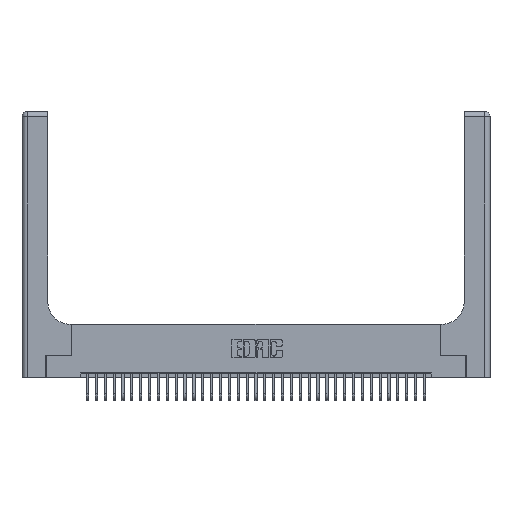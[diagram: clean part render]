
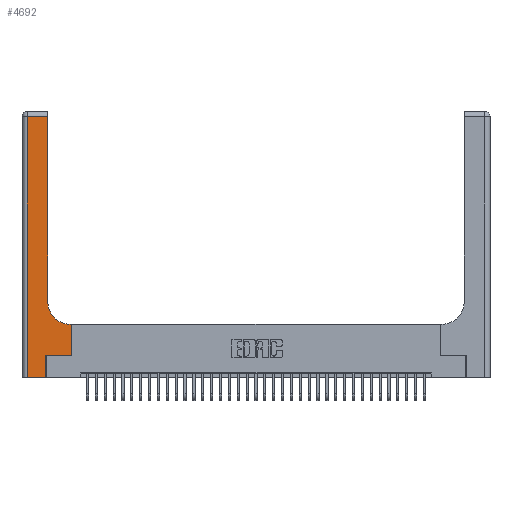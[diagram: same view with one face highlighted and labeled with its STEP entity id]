
A CAD part, top view. The second image highlights one B-rep face of the part: STEP entity #4692.
In plain terms, the highlighted planar face has unit normal (0, 0, 1).
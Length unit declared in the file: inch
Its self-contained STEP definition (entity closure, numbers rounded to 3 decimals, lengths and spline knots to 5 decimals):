
#306 = EDGE_CURVE ( 'NONE', #33902, #18627, #34485, .T. ) ;
#442 = ORIENTED_EDGE ( 'NONE', *, *, #20824, .T. ) ;
#2268 = DIRECTION ( 'NONE',  ( 0., 0., -1. ) ) ;
#2276 = VECTOR ( 'NONE', #25158, 39.37008 ) ;
#3361 = EDGE_CURVE ( 'NONE', #24542, #6409, #11562, .T. ) ;
#4110 = EDGE_CURVE ( 'NONE', #6556, #35407, #18662, .T. ) ;
#4316 = EDGE_CURVE ( 'NONE', #35407, #33902, #12256, .T. ) ;
#4446 = EDGE_CURVE ( 'NONE', #15794, #24542, #24082, .T. ) ;
#4692 = ADVANCED_FACE ( 'NONE', ( #30439 ), #23582, .F. ) ;
#5081 = CARTESIAN_POINT ( 'NONE',  ( 0., 0., 0.37 ) ) ;
#5613 = CARTESIAN_POINT ( 'NONE',  ( 0.5585, 0.6, 0.37 ) ) ;
#5939 = CARTESIAN_POINT ( 'NONE',  ( 0.2915, 2.94, 0.37 ) ) ;
#6409 = VERTEX_POINT ( 'NONE', #14225 ) ;
#6486 = CARTESIAN_POINT ( 'NONE',  ( 0., 2.94, 0.37 ) ) ;
#6556 = VERTEX_POINT ( 'NONE', #5939 ) ;
#7626 = LINE ( 'NONE', #31130, #37674 ) ;
#9256 = DIRECTION ( 'NONE',  ( -1., 0., 0. ) ) ;
#9596 = DIRECTION ( 'NONE',  ( -1., 0., 0. ) ) ;
#10860 = EDGE_CURVE ( 'NONE', #32946, #6556, #7626, .T. ) ;
#10862 = VECTOR ( 'NONE', #9596, 39.37008 ) ;
#11178 = VECTOR ( 'NONE', #35551, 39.37008 ) ;
#11288 = VECTOR ( 'NONE', #37239, 39.37008 ) ;
#11562 = LINE ( 'NONE', #29671, #33837 ) ;
#12000 = DIRECTION ( 'NONE',  ( -1., 0., 0. ) ) ;
#12256 = LINE ( 'NONE', #19156, #26821 ) ;
#14225 = CARTESIAN_POINT ( 'NONE',  ( 0.5415, 0.6, 0.37 ) ) ;
#15450 = VECTOR ( 'NONE', #31351, 39.37008 ) ;
#15794 = VERTEX_POINT ( 'NONE', #29598 ) ;
#16240 = DIRECTION ( 'NONE',  ( 0., -1., 0. ) ) ;
#18627 = VERTEX_POINT ( 'NONE', #32452 ) ;
#18662 = LINE ( 'NONE', #6486, #10862 ) ;
#18958 = LINE ( 'NONE', #32626, #11178 ) ;
#19156 = CARTESIAN_POINT ( 'NONE',  ( 0.06, 3., 0.37 ) ) ;
#19575 = DIRECTION ( 'NONE',  ( 0., 1., 0. ) ) ;
#19757 = ORIENTED_EDGE ( 'NONE', *, *, #10860, .T. ) ;
#19882 = CARTESIAN_POINT ( 'NONE',  ( 0.5415, 0.85, 0.37 ) ) ;
#20824 = EDGE_CURVE ( 'NONE', #6409, #32946, #32009, .T. ) ;
#21161 = ORIENTED_EDGE ( 'NONE', *, *, #4446, .T. ) ;
#22226 = CARTESIAN_POINT ( 'NONE',  ( 0.269, 0., 0.37 ) ) ;
#22479 = ORIENTED_EDGE ( 'NONE', *, *, #4316, .T. ) ;
#22786 = DIRECTION ( 'NONE',  ( 1., 0., 0. ) ) ;
#23582 = PLANE ( 'NONE',  #27340 ) ;
#24082 = LINE ( 'NONE', #34237, #15450 ) ;
#24542 = VERTEX_POINT ( 'NONE', #5613 ) ;
#24753 = LINE ( 'NONE', #22226, #2276 ) ;
#25158 = DIRECTION ( 'NONE',  ( 0., 1., 0. ) ) ;
#26515 = CARTESIAN_POINT ( 'NONE',  ( 0., 3., 0.37 ) ) ;
#26821 = VECTOR ( 'NONE', #16240, 39.37008 ) ;
#27340 = AXIS2_PLACEMENT_3D ( 'NONE', #26515, #29450, #12000 ) ;
#27902 = CARTESIAN_POINT ( 'NONE',  ( 0.06, 2.94, 0.37 ) ) ;
#28045 = EDGE_LOOP ( 'NONE', ( #19757, #35188, #22479, #30239, #32023, #35682, #21161, #30702, #442 ) ) ;
#29450 = DIRECTION ( 'NONE',  ( 0., 0., -1. ) ) ;
#29598 = CARTESIAN_POINT ( 'NONE',  ( 0.5585, 0.25, 0.37 ) ) ;
#29671 = CARTESIAN_POINT ( 'NONE',  ( 0.2915, 0.6, 0.37 ) ) ;
#30239 = ORIENTED_EDGE ( 'NONE', *, *, #306, .T. ) ;
#30439 = FACE_OUTER_BOUND ( 'NONE', #28045, .T. ) ;
#30520 = VERTEX_POINT ( 'NONE', #36344 ) ;
#30702 = ORIENTED_EDGE ( 'NONE', *, *, #3361, .T. ) ;
#31130 = CARTESIAN_POINT ( 'NONE',  ( 0.2915, 3., 0.37 ) ) ;
#31351 = DIRECTION ( 'NONE',  ( 0., 1., 0. ) ) ;
#32009 = CIRCLE ( 'NONE', #32590, 0.25 ) ;
#32023 = ORIENTED_EDGE ( 'NONE', *, *, #36049, .T. ) ;
#32149 = CARTESIAN_POINT ( 'NONE',  ( 0.06, 0., 0.37 ) ) ;
#32452 = CARTESIAN_POINT ( 'NONE',  ( 0.269, 0., 0.37 ) ) ;
#32590 = AXIS2_PLACEMENT_3D ( 'NONE', #19882, #2268, #22786 ) ;
#32626 = CARTESIAN_POINT ( 'NONE',  ( 0.269, 0.25, 0.37 ) ) ;
#32946 = VERTEX_POINT ( 'NONE', #35893 ) ;
#33837 = VECTOR ( 'NONE', #9256, 39.37008 ) ;
#33902 = VERTEX_POINT ( 'NONE', #32149 ) ;
#34237 = CARTESIAN_POINT ( 'NONE',  ( 0.5585, 0.25, 0.37 ) ) ;
#34485 = LINE ( 'NONE', #5081, #11288 ) ;
#34560 = EDGE_CURVE ( 'NONE', #30520, #15794, #18958, .T. ) ;
#35188 = ORIENTED_EDGE ( 'NONE', *, *, #4110, .T. ) ;
#35407 = VERTEX_POINT ( 'NONE', #27902 ) ;
#35551 = DIRECTION ( 'NONE',  ( 1., 0., 0. ) ) ;
#35682 = ORIENTED_EDGE ( 'NONE', *, *, #34560, .T. ) ;
#35893 = CARTESIAN_POINT ( 'NONE',  ( 0.2915, 0.85, 0.37 ) ) ;
#36049 = EDGE_CURVE ( 'NONE', #18627, #30520, #24753, .T. ) ;
#36344 = CARTESIAN_POINT ( 'NONE',  ( 0.269, 0.25, 0.37 ) ) ;
#37239 = DIRECTION ( 'NONE',  ( 1., 0., 0. ) ) ;
#37674 = VECTOR ( 'NONE', #19575, 39.37008 ) ;
